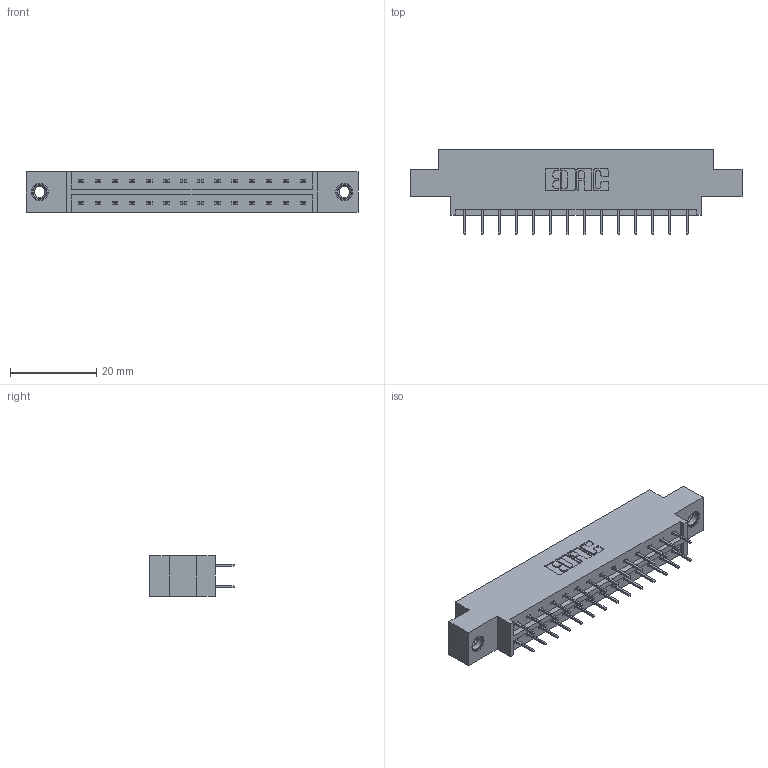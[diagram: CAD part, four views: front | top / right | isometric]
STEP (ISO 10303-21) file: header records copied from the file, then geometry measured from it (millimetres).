
FILE_DESCRIPTION (( 'STEP AP203' ), '1' );
FILE_NAME ('833-028-524-807.STEP', '2020-06-02T08:29:48', ( '' ), ( '' ), 'SwSTEP 2.0', 'SolidWorks 2020', '' );
FILE_SCHEMA (( 'CONFIG_CONTROL_DESIGN' ));
Length unit declared in the file: inch
Products named in the file (4): 345-250-001_345-250-005-103; 833-028-524-807; 833 Part_Offset - .156 Dia - TI; 345-292-001_345-293-124
Assembly tree (31 placements, depth 2):
  833-028-524-807
    833 Part_Offset - .156 Dia - TI
    345-292-001_345-293-124  x28
    345-250-001_345-250-005-103  x2
Bounding box: 77.01 x 19.69 x 9.4 mm (x, y, z)
Volume: 7317 mm3; surface area: 8477.5 mm2
Topology: 31 solids, 31 shells, 1746 faces, 4911 edges, 3154 vertices
Faces by surface type: plane 1282, cylinder 448, cone 12, torus 4
Entity records: 14020 total; most frequent: CARTESIAN_POINT 2341, ORIENTED_EDGE 2270, DIRECTION 2081, EDGE_CURVE 1135, VECTOR 991, LINE 991, VERTEX_POINT 748, AXIS2_PLACEMENT_3D 545
